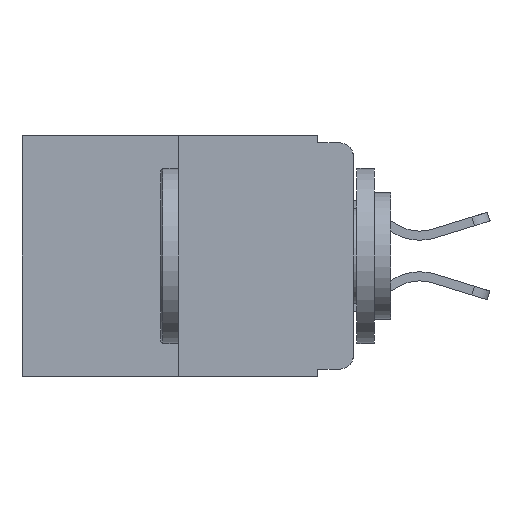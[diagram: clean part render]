
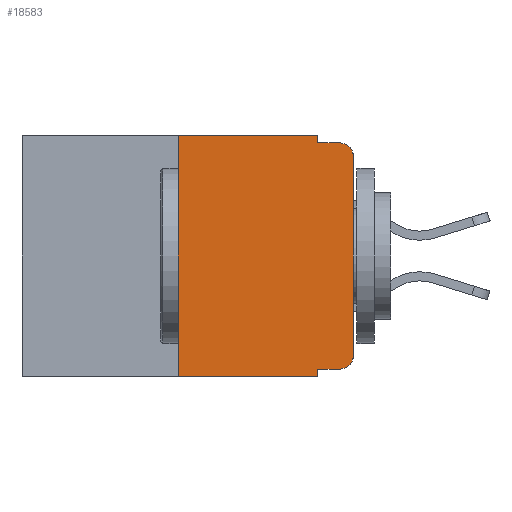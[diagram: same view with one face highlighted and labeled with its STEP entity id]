
A CAD part, left-side view. The second image highlights one B-rep face of the part: STEP entity #18583.
In plain terms, the highlighted planar face has unit normal (-1, 0, 0).
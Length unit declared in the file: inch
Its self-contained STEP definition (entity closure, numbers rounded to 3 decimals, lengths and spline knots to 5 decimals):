
#355 = VERTEX_POINT ( 'NONE', #5783 ) ;
#440 = CARTESIAN_POINT ( 'NONE',  ( 0., 0.051, -0.01 ) ) ;
#496 = EDGE_CURVE ( 'NONE', #23775, #20281, #2579, .T. ) ;
#1919 = DIRECTION ( 'NONE',  ( 0., -1., 0. ) ) ;
#1926 = EDGE_CURVE ( 'NONE', #355, #23775, #15833, .T. ) ;
#2034 = ORIENTED_EDGE ( 'NONE', *, *, #17620, .T. ) ;
#2115 = CARTESIAN_POINT ( 'NONE',  ( 0., 0.051, -0.333 ) ) ;
#2277 = LINE ( 'NONE', #2977, #7899 ) ;
#2579 = CIRCLE ( 'NONE', #14159, 0.02 ) ;
#2977 = CARTESIAN_POINT ( 'NONE',  ( 0., 0.051, 0. ) ) ;
#3245 = CARTESIAN_POINT ( 'NONE',  ( 0., 0.051, -0.01 ) ) ;
#3290 = EDGE_CURVE ( 'NONE', #355, #21381, #6895, .T. ) ;
#3323 = ORIENTED_EDGE ( 'NONE', *, *, #9531, .T. ) ;
#3877 = VERTEX_POINT ( 'NONE', #5255 ) ;
#4431 = FACE_OUTER_BOUND ( 'NONE', #18292, .T. ) ;
#4565 = EDGE_CURVE ( 'NONE', #9024, #3877, #8832, .T. ) ;
#4809 = VECTOR ( 'NONE', #9698, 39.37008 ) ;
#4977 = DIRECTION ( 'NONE',  ( 0., -1., 0. ) ) ;
#5095 = ORIENTED_EDGE ( 'NONE', *, *, #5827, .F. ) ;
#5255 = CARTESIAN_POINT ( 'NONE',  ( 0., 0.25, 0. ) ) ;
#5783 = CARTESIAN_POINT ( 'NONE',  ( 0., 0.051, -0.333 ) ) ;
#5827 = EDGE_CURVE ( 'NONE', #11615, #17686, #2277, .T. ) ;
#5906 = AXIS2_PLACEMENT_3D ( 'NONE', #17051, #7959, #20704 ) ;
#5923 = LINE ( 'NONE', #19948, #9648 ) ;
#6103 = PLANE ( 'NONE',  #5906 ) ;
#6182 = CARTESIAN_POINT ( 'NONE',  ( 0., 0., -0.313 ) ) ;
#6610 = CARTESIAN_POINT ( 'NONE',  ( 0., 0.051, 0. ) ) ;
#6624 = VECTOR ( 'NONE', #4977, 39.37008 ) ;
#6895 = LINE ( 'NONE', #6610, #11756 ) ;
#7054 = EDGE_CURVE ( 'NONE', #17686, #21863, #7199, .T. ) ;
#7119 = ORIENTED_EDGE ( 'NONE', *, *, #3290, .F. ) ;
#7199 = LINE ( 'NONE', #3245, #6624 ) ;
#7899 = VECTOR ( 'NONE', #15898, 39.37008 ) ;
#7959 = DIRECTION ( 'NONE',  ( 1., 0., 0. ) ) ;
#8027 = EDGE_CURVE ( 'NONE', #3877, #11615, #19999, .T. ) ;
#8106 = CARTESIAN_POINT ( 'NONE',  ( 0., 0., -0.03 ) ) ;
#8306 = EDGE_CURVE ( 'NONE', #17071, #21863, #9160, .T. ) ;
#8811 = VECTOR ( 'NONE', #11762, 39.37008 ) ;
#8832 = LINE ( 'NONE', #11169, #17961 ) ;
#9024 = VERTEX_POINT ( 'NONE', #22088 ) ;
#9160 = CIRCLE ( 'NONE', #9630, 0.02 ) ;
#9318 = DIRECTION ( 'NONE',  ( -1., 0., 0. ) ) ;
#9531 = EDGE_CURVE ( 'NONE', #20281, #17071, #5923, .T. ) ;
#9630 = AXIS2_PLACEMENT_3D ( 'NONE', #20235, #9318, #21973 ) ;
#9648 = VECTOR ( 'NONE', #21693, 39.37008 ) ;
#9698 = DIRECTION ( 'NONE',  ( 0., -1., 0. ) ) ;
#10426 = DIRECTION ( 'NONE',  ( 0., 0., -1. ) ) ;
#11169 = CARTESIAN_POINT ( 'NONE',  ( 0., 0.25, 0. ) ) ;
#11454 = CARTESIAN_POINT ( 'NONE',  ( 0., 0.473, 0. ) ) ;
#11527 = CARTESIAN_POINT ( 'NONE',  ( 0., 0.02, -0.333 ) ) ;
#11615 = VERTEX_POINT ( 'NONE', #12575 ) ;
#11756 = VECTOR ( 'NONE', #17618, 39.37008 ) ;
#11762 = DIRECTION ( 'NONE',  ( 0., -1., 0. ) ) ;
#12575 = CARTESIAN_POINT ( 'NONE',  ( 0., 0.051, 0. ) ) ;
#12832 = CARTESIAN_POINT ( 'NONE',  ( 0., 0.02, -0.01 ) ) ;
#13567 = CARTESIAN_POINT ( 'NONE',  ( 0., 0.473, -0.343 ) ) ;
#14159 = AXIS2_PLACEMENT_3D ( 'NONE', #21113, #21034, #10426 ) ;
#15275 = VECTOR ( 'NONE', #1919, 39.37008 ) ;
#15833 = LINE ( 'NONE', #2115, #15275 ) ;
#15898 = DIRECTION ( 'NONE',  ( 0., 0., -1. ) ) ;
#16023 = ORIENTED_EDGE ( 'NONE', *, *, #8027, .F. ) ;
#17051 = CARTESIAN_POINT ( 'NONE',  ( 0., 0.473, 0. ) ) ;
#17071 = VERTEX_POINT ( 'NONE', #8106 ) ;
#17618 = DIRECTION ( 'NONE',  ( 0., 0., -1. ) ) ;
#17620 = EDGE_CURVE ( 'NONE', #9024, #21381, #18524, .T. ) ;
#17686 = VERTEX_POINT ( 'NONE', #440 ) ;
#17961 = VECTOR ( 'NONE', #22006, 39.37008 ) ;
#18292 = EDGE_LOOP ( 'NONE', ( #3323, #22729, #18593, #5095, #16023, #20824, #2034, #7119, #21601, #22141 ) ) ;
#18524 = LINE ( 'NONE', #13567, #8811 ) ;
#18583 = ADVANCED_FACE ( 'NONE', ( #4431 ), #6103, .F. ) ;
#18593 = ORIENTED_EDGE ( 'NONE', *, *, #7054, .F. ) ;
#19948 = CARTESIAN_POINT ( 'NONE',  ( 0., 0., 0. ) ) ;
#19999 = LINE ( 'NONE', #11454, #4809 ) ;
#20235 = CARTESIAN_POINT ( 'NONE',  ( 0., 0.02, -0.03 ) ) ;
#20281 = VERTEX_POINT ( 'NONE', #6182 ) ;
#20618 = CARTESIAN_POINT ( 'NONE',  ( 0., 0.051, -0.343 ) ) ;
#20704 = DIRECTION ( 'NONE',  ( 0., 0., -1. ) ) ;
#20824 = ORIENTED_EDGE ( 'NONE', *, *, #4565, .F. ) ;
#21034 = DIRECTION ( 'NONE',  ( -1., 0., 0. ) ) ;
#21113 = CARTESIAN_POINT ( 'NONE',  ( 0., 0.02, -0.313 ) ) ;
#21381 = VERTEX_POINT ( 'NONE', #20618 ) ;
#21601 = ORIENTED_EDGE ( 'NONE', *, *, #1926, .T. ) ;
#21693 = DIRECTION ( 'NONE',  ( 0., 0., 1. ) ) ;
#21863 = VERTEX_POINT ( 'NONE', #12832 ) ;
#21973 = DIRECTION ( 'NONE',  ( 0., 0., -1. ) ) ;
#22006 = DIRECTION ( 'NONE',  ( 0., 0., 1. ) ) ;
#22088 = CARTESIAN_POINT ( 'NONE',  ( 0., 0.25, -0.343 ) ) ;
#22141 = ORIENTED_EDGE ( 'NONE', *, *, #496, .T. ) ;
#22729 = ORIENTED_EDGE ( 'NONE', *, *, #8306, .T. ) ;
#23775 = VERTEX_POINT ( 'NONE', #11527 ) ;
